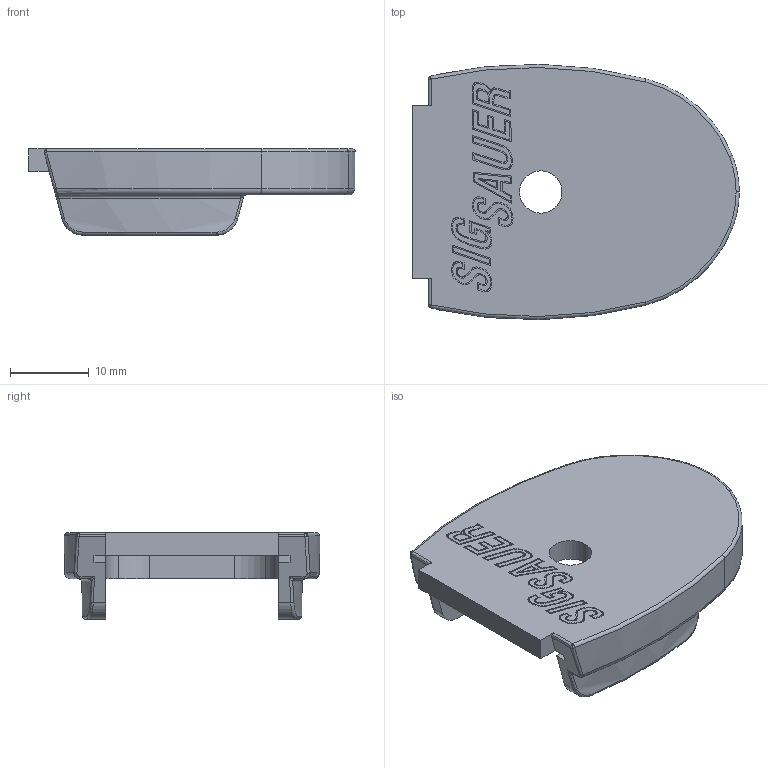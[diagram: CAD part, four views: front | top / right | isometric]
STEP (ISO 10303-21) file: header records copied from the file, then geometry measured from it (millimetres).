
FILE_DESCRIPTION (( 'STEP AP214' ), '1' );
FILE_NAME ('Magazine Floorplate.step', '2014-07-30T19:46:11', ( 'WarFairy' ), ( '' ), 'SwSTEP 2.0', 'SolidWorks 2013', '' );
FILE_SCHEMA (( 'AUTOMOTIVE_DESIGN' ));
Length unit declared in the file: millimetre
Products named in the file (1): Magazine Floorplate
Bounding box: 41.54 x 32.48 x 10.99 mm (x, y, z)
Volume: 5034.6 mm3; surface area: 3886.4 mm2
Topology: 1 solids, 1 shells, 355 faces, 963 edges, 628 vertices
Faces by surface type: plane 182, bspline 121, cylinder 33, torus 15, sphere 4
Entity records: 12056 total; most frequent: CARTESIAN_POINT 3944, ORIENTED_EDGE 1922, DIRECTION 1230, EDGE_CURVE 961, VERTEX_POINT 628, VECTOR 610, LINE 610, EDGE_LOOP 377
